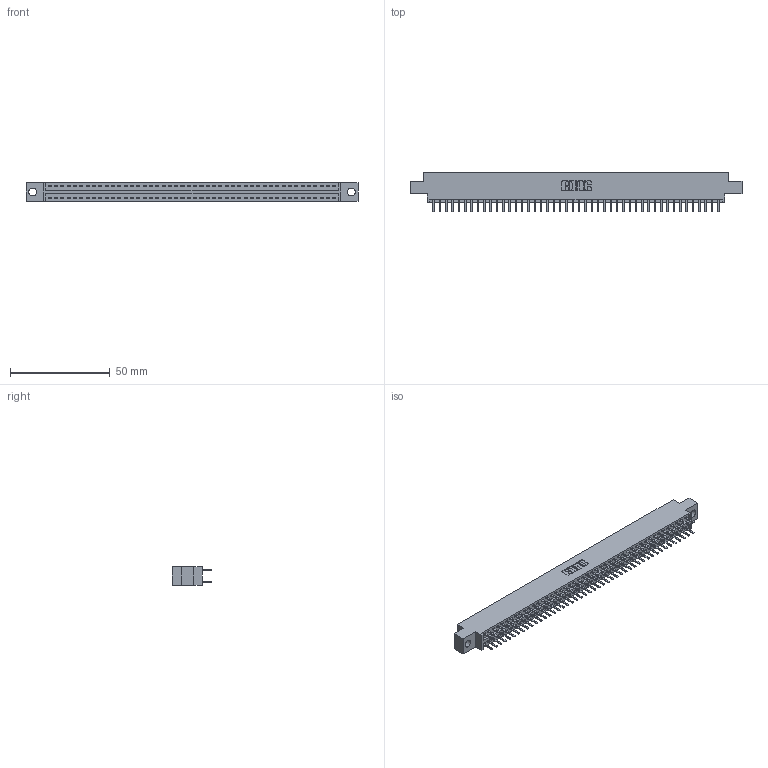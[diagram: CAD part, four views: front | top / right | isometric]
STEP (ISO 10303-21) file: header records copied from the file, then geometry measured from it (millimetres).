
FILE_DESCRIPTION (( 'STEP AP203' ), '1' );
FILE_NAME ('346-092-520-804.STEP', '2018-08-30T03:00:15', ( '' ), ( '' ), 'SwSTEP 2.0', 'SolidWorks 2016', '' );
FILE_SCHEMA (( 'CONFIG_CONTROL_DESIGN' ));
Length unit declared in the file: inch
Products named in the file (3): 345-292-001_345-293-120; 346-092-520-804; 346 Part_0.170 Offset - 0.156 Dia-TH
Assembly tree (93 placements, depth 2):
  346-092-520-804
    346 Part_0.170 Offset - 0.156 Dia-TH
    345-292-001_345-293-120  x92
Bounding box: 166.62 x 20.02 x 9.4 mm (x, y, z)
Volume: 15996.1 mm3; surface area: 21948.7 mm2
Topology: 93 solids, 93 shells, 5278 faces, 15337 edges, 9978 vertices
Faces by surface type: plane 3484, cylinder 1794
Entity records: 29731 total; most frequent: CARTESIAN_POINT 4908, ORIENTED_EDGE 4830, DIRECTION 4363, EDGE_CURVE 2415, LINE 2095, VECTOR 2095, VERTEX_POINT 1606, AXIS2_PLACEMENT_3D 1134
